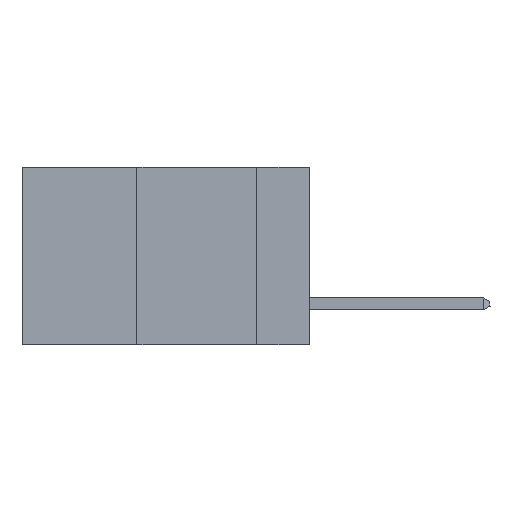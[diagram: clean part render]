
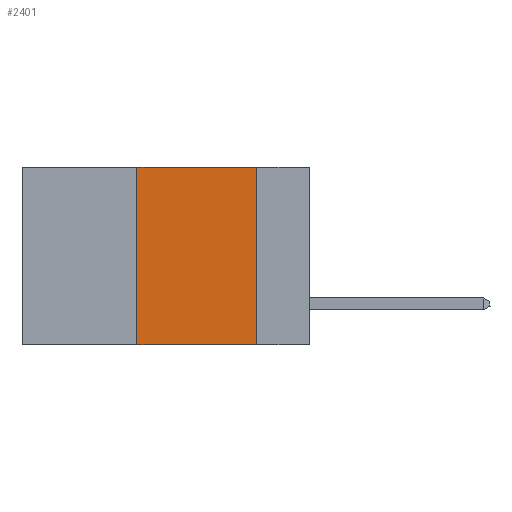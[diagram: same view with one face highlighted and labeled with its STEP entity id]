
A CAD part, left-side view. The second image highlights one B-rep face of the part: STEP entity #2401.
In plain terms, the highlighted planar face has unit normal (-1, 0, 0).
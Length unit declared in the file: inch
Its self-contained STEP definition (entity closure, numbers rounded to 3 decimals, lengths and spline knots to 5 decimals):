
#328 = VECTOR ( 'NONE', #8662, 39.37008 ) ;
#418 = EDGE_CURVE ( 'NONE', #1071, #9294, #7147, .T. ) ;
#488 = DIRECTION ( 'NONE',  ( 0., -1., 0. ) ) ;
#1008 = PLANE ( 'NONE',  #8532 ) ;
#1071 = VERTEX_POINT ( 'NONE', #3675 ) ;
#1081 = ORIENTED_EDGE ( 'NONE', *, *, #5551, .T. ) ;
#1321 = LINE ( 'NONE', #3492, #3799 ) ;
#1800 = VERTEX_POINT ( 'NONE', #1896 ) ;
#1896 = CARTESIAN_POINT ( 'NONE',  ( 0., 0.36, -0.37 ) ) ;
#2401 = ADVANCED_FACE ( 'NONE', ( #10535 ), #1008, .F. ) ;
#2797 = EDGE_CURVE ( 'NONE', #9294, #4440, #1321, .T. ) ;
#2829 = ORIENTED_EDGE ( 'NONE', *, *, #2797, .F. ) ;
#2935 = CARTESIAN_POINT ( 'NONE',  ( 0., 0.6, 0. ) ) ;
#2945 = LINE ( 'NONE', #10273, #328 ) ;
#3044 = DIRECTION ( 'NONE',  ( 1., 0., 0. ) ) ;
#3492 = CARTESIAN_POINT ( 'NONE',  ( 0., 0.11, 0. ) ) ;
#3675 = CARTESIAN_POINT ( 'NONE',  ( 0., 0.36, 0. ) ) ;
#3799 = VECTOR ( 'NONE', #9283, 39.37008 ) ;
#4012 = CARTESIAN_POINT ( 'NONE',  ( 0., 0.11, -0.37 ) ) ;
#4092 = CARTESIAN_POINT ( 'NONE',  ( 0., 0.36, 0. ) ) ;
#4440 = VERTEX_POINT ( 'NONE', #4012 ) ;
#4484 = ORIENTED_EDGE ( 'NONE', *, *, #418, .F. ) ;
#4666 = DIRECTION ( 'NONE',  ( 0., 0., -1. ) ) ;
#5551 = EDGE_CURVE ( 'NONE', #1800, #4440, #2945, .T. ) ;
#6101 = ORIENTED_EDGE ( 'NONE', *, *, #8814, .F. ) ;
#6612 = CARTESIAN_POINT ( 'NONE',  ( 0., 0.11, 0. ) ) ;
#7147 = LINE ( 'NONE', #7849, #10260 ) ;
#7421 = DIRECTION ( 'NONE',  ( 0., 0., 1. ) ) ;
#7849 = CARTESIAN_POINT ( 'NONE',  ( 0., 0.6, 0. ) ) ;
#8532 = AXIS2_PLACEMENT_3D ( 'NONE', #2935, #3044, #4666 ) ;
#8662 = DIRECTION ( 'NONE',  ( 0., -1., 0. ) ) ;
#8681 = VECTOR ( 'NONE', #7421, 39.37008 ) ;
#8814 = EDGE_CURVE ( 'NONE', #1800, #1071, #9852, .T. ) ;
#9283 = DIRECTION ( 'NONE',  ( 0., 0., -1. ) ) ;
#9294 = VERTEX_POINT ( 'NONE', #6612 ) ;
#9852 = LINE ( 'NONE', #4092, #8681 ) ;
#9856 = EDGE_LOOP ( 'NONE', ( #2829, #4484, #6101, #1081 ) ) ;
#10260 = VECTOR ( 'NONE', #488, 39.37008 ) ;
#10273 = CARTESIAN_POINT ( 'NONE',  ( 0., 0.6, -0.37 ) ) ;
#10535 = FACE_OUTER_BOUND ( 'NONE', #9856, .T. ) ;
